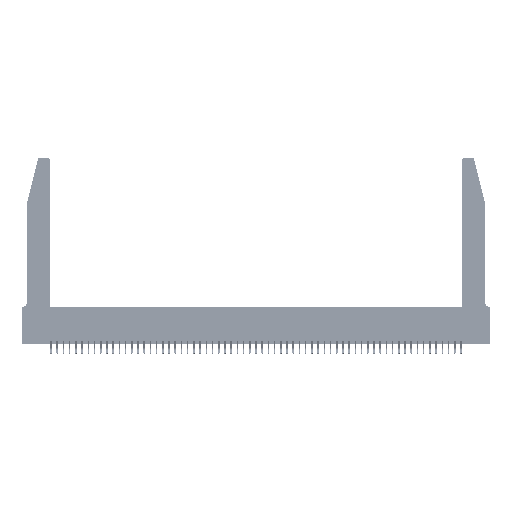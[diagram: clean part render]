
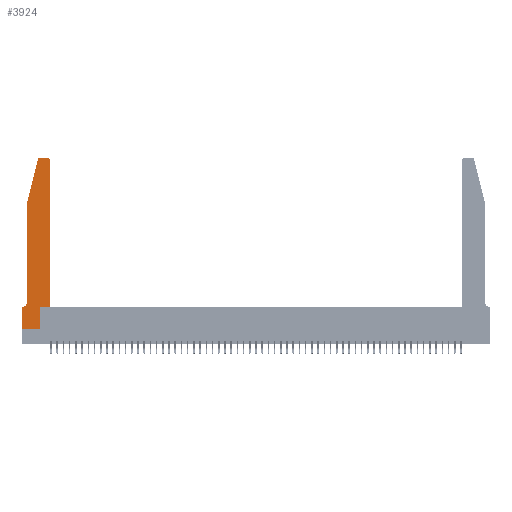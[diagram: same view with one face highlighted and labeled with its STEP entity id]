
A CAD part, top view. The second image highlights one B-rep face of the part: STEP entity #3924.
In plain terms, the highlighted planar face has unit normal (0, 0, 1).
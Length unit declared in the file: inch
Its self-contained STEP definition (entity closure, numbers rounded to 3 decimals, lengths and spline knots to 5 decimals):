
#244 = CARTESIAN_POINT ( 'NONE',  ( 0.4505, 0.35, 0.37 ) ) ;
#672 = VECTOR ( 'NONE', #45400, 39.37008 ) ;
#1020 = LINE ( 'NONE', #43346, #10184 ) ;
#1571 = CARTESIAN_POINT ( 'NONE',  ( 0.284, 2.72, 0.37 ) ) ;
#1729 = ORIENTED_EDGE ( 'NONE', *, *, #48682, .T. ) ;
#1859 = CARTESIAN_POINT ( 'NONE',  ( 0., 0.35, 0.37 ) ) ;
#1928 = CARTESIAN_POINT ( 'NONE',  ( 0.0755, 0.35, 0.37 ) ) ;
#2088 = EDGE_CURVE ( 'NONE', #4603, #25495, #6147, .T. ) ;
#2197 = CARTESIAN_POINT ( 'NONE',  ( 0.0755, 2., 0.37 ) ) ;
#2379 = AXIS2_PLACEMENT_3D ( 'NONE', #1571, #13795, #34621 ) ;
#3868 = CARTESIAN_POINT ( 'NONE',  ( 0.4505, 0.35, 0.37 ) ) ;
#3924 = ADVANCED_FACE ( 'NONE', ( #15134 ), #10059, .T. ) ;
#3926 = LINE ( 'NONE', #18880, #42575 ) ;
#4603 = VERTEX_POINT ( 'NONE', #17829 ) ;
#5107 = EDGE_CURVE ( 'NONE', #24044, #28871, #53039, .T. ) ;
#6147 = CIRCLE ( 'NONE', #19077, 0.03 ) ;
#7665 = EDGE_CURVE ( 'NONE', #47200, #14292, #18087, .T. ) ;
#7981 = CARTESIAN_POINT ( 'NONE',  ( 0.0755, 2., 0.37 ) ) ;
#8200 = CARTESIAN_POINT ( 'NONE',  ( 0., 0., 0.37 ) ) ;
#10059 = PLANE ( 'NONE',  #36307 ) ;
#10184 = VECTOR ( 'NONE', #47356, 39.37008 ) ;
#11763 = EDGE_CURVE ( 'NONE', #25495, #24044, #32705, .T. ) ;
#11965 = VECTOR ( 'NONE', #21570, 39.37008 ) ;
#12184 = CARTESIAN_POINT ( 'NONE',  ( 0.4205, 2.72, 0.37 ) ) ;
#13350 = EDGE_CURVE ( 'NONE', #40983, #4603, #3926, .T. ) ;
#13430 = ORIENTED_EDGE ( 'NONE', *, *, #14681, .T. ) ;
#13702 = LINE ( 'NONE', #3868, #53040 ) ;
#13795 = DIRECTION ( 'NONE',  ( 0., 0., 1. ) ) ;
#14292 = VERTEX_POINT ( 'NONE', #8200 ) ;
#14449 = DIRECTION ( 'NONE',  ( 1., 0., 0. ) ) ;
#14681 = EDGE_CURVE ( 'NONE', #44957, #41695, #48272, .T. ) ;
#14778 = EDGE_LOOP ( 'NONE', ( #42642, #51259, #53728, #32917, #1729, #25127, #30199, #37467, #13430, #46670, #17068, #37578 ) ) ;
#15134 = FACE_OUTER_BOUND ( 'NONE', #14778, .T. ) ;
#15772 = DIRECTION ( 'NONE',  ( 0., 1., 0. ) ) ;
#17035 = CARTESIAN_POINT ( 'NONE',  ( 0.25487, 2.72718, 0.37 ) ) ;
#17068 = ORIENTED_EDGE ( 'NONE', *, *, #13350, .T. ) ;
#17291 = CARTESIAN_POINT ( 'NONE',  ( 0.2865, 0.35, 0.37 ) ) ;
#17829 = CARTESIAN_POINT ( 'NONE',  ( 0.4505, 2.72, 0.37 ) ) ;
#18087 = LINE ( 'NONE', #37560, #47578 ) ;
#18398 = VERTEX_POINT ( 'NONE', #29470 ) ;
#18880 = CARTESIAN_POINT ( 'NONE',  ( 0.4505, 0.35, 0.37 ) ) ;
#19077 = AXIS2_PLACEMENT_3D ( 'NONE', #12184, #33389, #33204 ) ;
#19465 = DIRECTION ( 'NONE',  ( 0., 1., 0. ) ) ;
#21500 = VECTOR ( 'NONE', #43973, 39.37008 ) ;
#21570 = DIRECTION ( 'NONE',  ( 0., -1., 0. ) ) ;
#22917 = DIRECTION ( 'NONE',  ( -1., 0., 0. ) ) ;
#23816 = EDGE_CURVE ( 'NONE', #41695, #40983, #13702, .T. ) ;
#24044 = VERTEX_POINT ( 'NONE', #34704 ) ;
#25081 = DIRECTION ( 'NONE',  ( 0., -1., 0. ) ) ;
#25127 = ORIENTED_EDGE ( 'NONE', *, *, #31241, .T. ) ;
#25495 = VERTEX_POINT ( 'NONE', #40624 ) ;
#27716 = EDGE_CURVE ( 'NONE', #14292, #44957, #1020, .T. ) ;
#27725 = VERTEX_POINT ( 'NONE', #39475 ) ;
#28871 = VERTEX_POINT ( 'NONE', #17035 ) ;
#29470 = CARTESIAN_POINT ( 'NONE',  ( 0.0755, 0.42, 0.37 ) ) ;
#29718 = VERTEX_POINT ( 'NONE', #2197 ) ;
#30199 = ORIENTED_EDGE ( 'NONE', *, *, #7665, .T. ) ;
#30381 = CARTESIAN_POINT ( 'NONE',  ( 0., 0.35, 0.37 ) ) ;
#31218 = CARTESIAN_POINT ( 'NONE',  ( 0.2865, 0.35, 0.37 ) ) ;
#31241 = EDGE_CURVE ( 'NONE', #27725, #47200, #47735, .T. ) ;
#32567 = VECTOR ( 'NONE', #19465, 39.37008 ) ;
#32705 = LINE ( 'NONE', #36764, #672 ) ;
#32917 = ORIENTED_EDGE ( 'NONE', *, *, #33623, .T. ) ;
#33193 = DIRECTION ( 'NONE',  ( -0.239, -0.971, 0. ) ) ;
#33204 = DIRECTION ( 'NONE',  ( 1., 0., 0. ) ) ;
#33389 = DIRECTION ( 'NONE',  ( 0., 0., 1. ) ) ;
#33623 = EDGE_CURVE ( 'NONE', #29718, #18398, #45991, .T. ) ;
#34217 = CARTESIAN_POINT ( 'NONE',  ( 0.0755, 2., 0.37 ) ) ;
#34621 = DIRECTION ( 'NONE',  ( 1., 0., 0. ) ) ;
#34704 = CARTESIAN_POINT ( 'NONE',  ( 0.284, 2.75, 0.37 ) ) ;
#34885 = CARTESIAN_POINT ( 'NONE',  ( 0.2865, 0., 0.37 ) ) ;
#35290 = DIRECTION ( 'NONE',  ( 0., 0., 1. ) ) ;
#36307 = AXIS2_PLACEMENT_3D ( 'NONE', #1859, #35290, #14449 ) ;
#36549 = LINE ( 'NONE', #7981, #49657 ) ;
#36764 = CARTESIAN_POINT ( 'NONE',  ( 0.2605, 2.75, 0.37 ) ) ;
#37420 = AXIS2_PLACEMENT_3D ( 'NONE', #39771, #44169, #22917 ) ;
#37467 = ORIENTED_EDGE ( 'NONE', *, *, #27716, .T. ) ;
#37560 = CARTESIAN_POINT ( 'NONE',  ( 0., 0., 0.37 ) ) ;
#37578 = ORIENTED_EDGE ( 'NONE', *, *, #2088, .T. ) ;
#39475 = CARTESIAN_POINT ( 'NONE',  ( 0.0055, 0.35, 0.37 ) ) ;
#39771 = CARTESIAN_POINT ( 'NONE',  ( 0.0055, 0.42, 0.37 ) ) ;
#40624 = CARTESIAN_POINT ( 'NONE',  ( 0.4205, 2.75, 0.37 ) ) ;
#40983 = VERTEX_POINT ( 'NONE', #244 ) ;
#41695 = VERTEX_POINT ( 'NONE', #17291 ) ;
#42575 = VECTOR ( 'NONE', #15772, 39.37008 ) ;
#42642 = ORIENTED_EDGE ( 'NONE', *, *, #11763, .T. ) ;
#43346 = CARTESIAN_POINT ( 'NONE',  ( 0., 0., 0.37 ) ) ;
#43568 = EDGE_CURVE ( 'NONE', #28871, #29718, #36549, .T. ) ;
#43973 = DIRECTION ( 'NONE',  ( -1., 0., 0. ) ) ;
#44169 = DIRECTION ( 'NONE',  ( 0., 0., -1. ) ) ;
#44957 = VERTEX_POINT ( 'NONE', #34885 ) ;
#45400 = DIRECTION ( 'NONE',  ( -1., 0., 0. ) ) ;
#45991 = LINE ( 'NONE', #34217, #11965 ) ;
#46670 = ORIENTED_EDGE ( 'NONE', *, *, #23816, .T. ) ;
#47078 = CIRCLE ( 'NONE', #37420, 0.07 ) ;
#47200 = VERTEX_POINT ( 'NONE', #30381 ) ;
#47356 = DIRECTION ( 'NONE',  ( 1., 0., 0. ) ) ;
#47578 = VECTOR ( 'NONE', #25081, 39.37008 ) ;
#47735 = LINE ( 'NONE', #1928, #21500 ) ;
#48272 = LINE ( 'NONE', #31218, #32567 ) ;
#48682 = EDGE_CURVE ( 'NONE', #18398, #27725, #47078, .T. ) ;
#49600 = DIRECTION ( 'NONE',  ( 1., 0., 0. ) ) ;
#49657 = VECTOR ( 'NONE', #33193, 39.37008 ) ;
#51259 = ORIENTED_EDGE ( 'NONE', *, *, #5107, .T. ) ;
#53039 = CIRCLE ( 'NONE', #2379, 0.03 ) ;
#53040 = VECTOR ( 'NONE', #49600, 39.37008 ) ;
#53728 = ORIENTED_EDGE ( 'NONE', *, *, #43568, .T. ) ;
